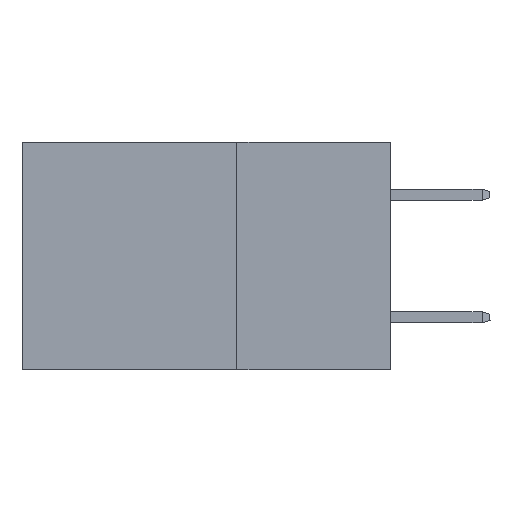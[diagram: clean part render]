
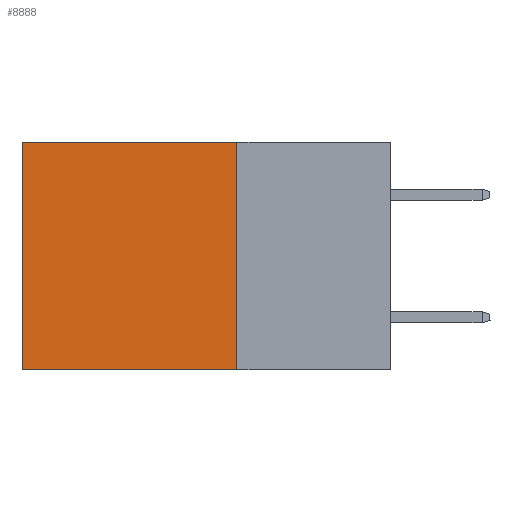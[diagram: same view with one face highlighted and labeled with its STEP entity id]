
A CAD part, left-side view. The second image highlights one B-rep face of the part: STEP entity #8888.
In plain terms, the highlighted planar face has unit normal (-1, 0, 0).
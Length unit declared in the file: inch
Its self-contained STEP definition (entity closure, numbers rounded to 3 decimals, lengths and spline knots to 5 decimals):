
#717 = DIRECTION ( 'NONE',  ( 0., 0., -1. ) ) ;
#1363 = ORIENTED_EDGE ( 'NONE', *, *, #13526, .T. ) ;
#1626 = DIRECTION ( 'NONE',  ( 1., 0., 0. ) ) ;
#1686 = DIRECTION ( 'NONE',  ( 0., 0., -1. ) ) ;
#2201 = DIRECTION ( 'NONE',  ( 0., 0., -1. ) ) ;
#2349 = VECTOR ( 'NONE', #717, 39.37008 ) ;
#2446 = VERTEX_POINT ( 'NONE', #17986 ) ;
#3639 = DIRECTION ( 'NONE',  ( 0., 1., 0. ) ) ;
#3776 = EDGE_CURVE ( 'NONE', #2446, #15825, #13233, .T. ) ;
#3795 = VERTEX_POINT ( 'NONE', #20123 ) ;
#4377 = VECTOR ( 'NONE', #7757, 39.37008 ) ;
#4468 = CARTESIAN_POINT ( 'NONE',  ( 0.2875, 0.6, 0. ) ) ;
#5570 = CARTESIAN_POINT ( 'NONE',  ( 0.2875, 0.25, 0. ) ) ;
#5773 = AXIS2_PLACEMENT_3D ( 'NONE', #16420, #1626, #1686 ) ;
#5855 = LINE ( 'NONE', #16787, #21001 ) ;
#6119 = VERTEX_POINT ( 'NONE', #4468 ) ;
#6479 = LINE ( 'NONE', #20578, #4377 ) ;
#7757 = DIRECTION ( 'NONE',  ( 0., 1., 0. ) ) ;
#8888 = ADVANCED_FACE ( 'NONE', ( #18480 ), #11625, .F. ) ;
#9947 = ORIENTED_EDGE ( 'NONE', *, *, #11230, .T. ) ;
#10322 = CARTESIAN_POINT ( 'NONE',  ( 0.2875, 0.25, -0.37 ) ) ;
#10468 = VECTOR ( 'NONE', #3639, 39.37008 ) ;
#10895 = EDGE_CURVE ( 'NONE', #3795, #2446, #15939, .T. ) ;
#11230 = EDGE_CURVE ( 'NONE', #3795, #6119, #6479, .T. ) ;
#11625 = PLANE ( 'NONE',  #5773 ) ;
#13233 = LINE ( 'NONE', #10322, #10468 ) ;
#13445 = ORIENTED_EDGE ( 'NONE', *, *, #3776, .F. ) ;
#13526 = EDGE_CURVE ( 'NONE', #6119, #15825, #5855, .T. ) ;
#15468 = EDGE_LOOP ( 'NONE', ( #1363, #13445, #18496, #9947 ) ) ;
#15825 = VERTEX_POINT ( 'NONE', #19333 ) ;
#15939 = LINE ( 'NONE', #5570, #2349 ) ;
#16420 = CARTESIAN_POINT ( 'NONE',  ( 0.2875, 0.25, 0. ) ) ;
#16787 = CARTESIAN_POINT ( 'NONE',  ( 0.2875, 0.6, 0. ) ) ;
#17986 = CARTESIAN_POINT ( 'NONE',  ( 0.2875, 0.25, -0.37 ) ) ;
#18480 = FACE_OUTER_BOUND ( 'NONE', #15468, .T. ) ;
#18496 = ORIENTED_EDGE ( 'NONE', *, *, #10895, .F. ) ;
#19333 = CARTESIAN_POINT ( 'NONE',  ( 0.2875, 0.6, -0.37 ) ) ;
#20123 = CARTESIAN_POINT ( 'NONE',  ( 0.2875, 0.25, 0. ) ) ;
#20578 = CARTESIAN_POINT ( 'NONE',  ( 0.2875, 0.25, 0. ) ) ;
#21001 = VECTOR ( 'NONE', #2201, 39.37008 ) ;
